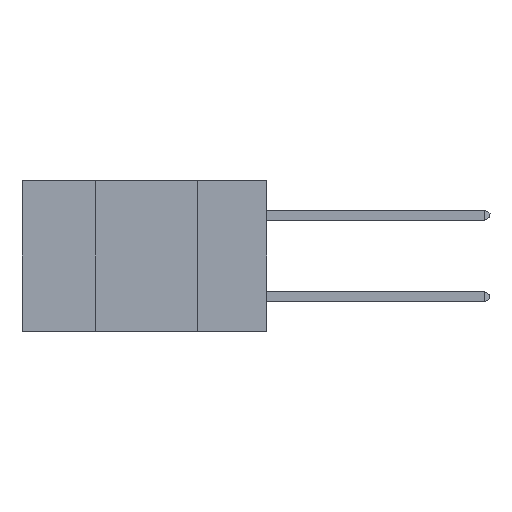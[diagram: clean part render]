
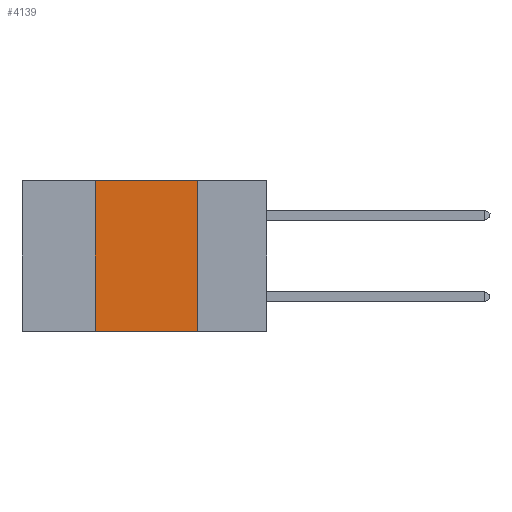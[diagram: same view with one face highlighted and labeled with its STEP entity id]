
A CAD part, left-side view. The second image highlights one B-rep face of the part: STEP entity #4139.
In plain terms, the highlighted planar face has unit normal (-1, 0, 0).
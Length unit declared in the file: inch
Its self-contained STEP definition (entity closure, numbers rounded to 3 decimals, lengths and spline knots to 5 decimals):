
#14 = FACE_OUTER_BOUND ( 'NONE', #12717, .T. ) ;
#1279 = ORIENTED_EDGE ( 'NONE', *, *, #6585, .T. ) ;
#2227 = VERTEX_POINT ( 'NONE', #10305 ) ;
#2556 = ORIENTED_EDGE ( 'NONE', *, *, #5395, .F. ) ;
#2578 = CARTESIAN_POINT ( 'NONE',  ( 0., 0.42, -0.37 ) ) ;
#3985 = CARTESIAN_POINT ( 'NONE',  ( 0., 0.17, 0. ) ) ;
#4139 = ADVANCED_FACE ( 'NONE', ( #14 ), #6226, .F. ) ;
#4493 = DIRECTION ( 'NONE',  ( 0., 0., -1. ) ) ;
#5395 = EDGE_CURVE ( 'NONE', #9496, #8146, #6446, .T. ) ;
#5597 = DIRECTION ( 'NONE',  ( 1., 0., 0. ) ) ;
#6203 = DIRECTION ( 'NONE',  ( 0., -1., 0. ) ) ;
#6226 = PLANE ( 'NONE',  #8821 ) ;
#6237 = LINE ( 'NONE', #9464, #8443 ) ;
#6446 = LINE ( 'NONE', #11630, #7975 ) ;
#6559 = EDGE_CURVE ( 'NONE', #8146, #2227, #9115, .T. ) ;
#6585 = EDGE_CURVE ( 'NONE', #9496, #9654, #6237, .T. ) ;
#7099 = ORIENTED_EDGE ( 'NONE', *, *, #6559, .F. ) ;
#7864 = CARTESIAN_POINT ( 'NONE',  ( 0., 0.6, 0. ) ) ;
#7975 = VECTOR ( 'NONE', #11696, 39.37008 ) ;
#8069 = VECTOR ( 'NONE', #13700, 39.37008 ) ;
#8093 = ORIENTED_EDGE ( 'NONE', *, *, #8572, .F. ) ;
#8146 = VERTEX_POINT ( 'NONE', #8910 ) ;
#8401 = LINE ( 'NONE', #3985, #8069 ) ;
#8443 = VECTOR ( 'NONE', #11572, 39.37008 ) ;
#8572 = EDGE_CURVE ( 'NONE', #2227, #9654, #8401, .T. ) ;
#8821 = AXIS2_PLACEMENT_3D ( 'NONE', #7864, #5597, #4493 ) ;
#8910 = CARTESIAN_POINT ( 'NONE',  ( 0., 0.42, 0. ) ) ;
#9115 = LINE ( 'NONE', #12556, #11580 ) ;
#9464 = CARTESIAN_POINT ( 'NONE',  ( 0., 0.6, -0.37 ) ) ;
#9496 = VERTEX_POINT ( 'NONE', #2578 ) ;
#9543 = CARTESIAN_POINT ( 'NONE',  ( 0., 0.17, -0.37 ) ) ;
#9654 = VERTEX_POINT ( 'NONE', #9543 ) ;
#10305 = CARTESIAN_POINT ( 'NONE',  ( 0., 0.17, 0. ) ) ;
#11572 = DIRECTION ( 'NONE',  ( 0., -1., 0. ) ) ;
#11580 = VECTOR ( 'NONE', #6203, 39.37008 ) ;
#11630 = CARTESIAN_POINT ( 'NONE',  ( 0., 0.42, 0. ) ) ;
#11696 = DIRECTION ( 'NONE',  ( 0., 0., 1. ) ) ;
#12556 = CARTESIAN_POINT ( 'NONE',  ( 0., 0.6, 0. ) ) ;
#12717 = EDGE_LOOP ( 'NONE', ( #8093, #7099, #2556, #1279 ) ) ;
#13700 = DIRECTION ( 'NONE',  ( 0., 0., -1. ) ) ;
